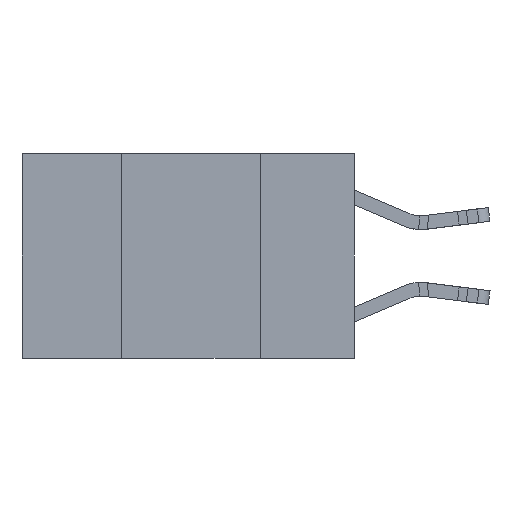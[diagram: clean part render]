
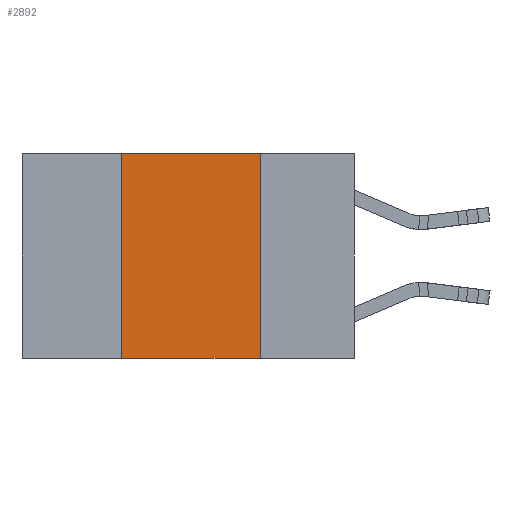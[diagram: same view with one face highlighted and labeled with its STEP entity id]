
A CAD part, left-side view. The second image highlights one B-rep face of the part: STEP entity #2892.
In plain terms, the highlighted planar face has unit normal (-1, 0, 0).
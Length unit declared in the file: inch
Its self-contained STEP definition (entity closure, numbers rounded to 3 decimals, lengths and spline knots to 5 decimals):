
#360 = LINE ( 'NONE', #27337, #17526 ) ;
#575 = LINE ( 'NONE', #24805, #24585 ) ;
#796 = CARTESIAN_POINT ( 'NONE',  ( 0., 0.17, -0.37 ) ) ;
#975 = VERTEX_POINT ( 'NONE', #23455 ) ;
#1849 = DIRECTION ( 'NONE',  ( 0., -1., 0. ) ) ;
#1882 = AXIS2_PLACEMENT_3D ( 'NONE', #5179, #29507, #25401 ) ;
#2091 = DIRECTION ( 'NONE',  ( 0., 0., 1. ) ) ;
#2797 = DIRECTION ( 'NONE',  ( 0., 0., -1. ) ) ;
#2892 = ADVANCED_FACE ( 'NONE', ( #9422 ), #16339, .F. ) ;
#4209 = VECTOR ( 'NONE', #2797, 39.37008 ) ;
#4938 = LINE ( 'NONE', #5196, #4209 ) ;
#5125 = CARTESIAN_POINT ( 'NONE',  ( 0., 0.17, 0. ) ) ;
#5179 = CARTESIAN_POINT ( 'NONE',  ( 0., 0.6, 0. ) ) ;
#5196 = CARTESIAN_POINT ( 'NONE',  ( 0., 0.17, 0. ) ) ;
#8936 = VERTEX_POINT ( 'NONE', #5125 ) ;
#9033 = VERTEX_POINT ( 'NONE', #796 ) ;
#9422 = FACE_OUTER_BOUND ( 'NONE', #16592, .T. ) ;
#9629 = EDGE_CURVE ( 'NONE', #8936, #9033, #4938, .T. ) ;
#10108 = ORIENTED_EDGE ( 'NONE', *, *, #12278, .F. ) ;
#12278 = EDGE_CURVE ( 'NONE', #975, #22771, #14289, .T. ) ;
#13565 = VECTOR ( 'NONE', #2091, 39.37008 ) ;
#13722 = ORIENTED_EDGE ( 'NONE', *, *, #23554, .F. ) ;
#13771 = CARTESIAN_POINT ( 'NONE',  ( 0., 0.42, 0. ) ) ;
#14289 = LINE ( 'NONE', #13771, #13565 ) ;
#16339 = PLANE ( 'NONE',  #1882 ) ;
#16592 = EDGE_LOOP ( 'NONE', ( #21715, #13722, #10108, #26394 ) ) ;
#17526 = VECTOR ( 'NONE', #1849, 39.37008 ) ;
#20168 = EDGE_CURVE ( 'NONE', #975, #9033, #575, .T. ) ;
#21715 = ORIENTED_EDGE ( 'NONE', *, *, #9629, .F. ) ;
#22771 = VERTEX_POINT ( 'NONE', #28849 ) ;
#23455 = CARTESIAN_POINT ( 'NONE',  ( 0., 0.42, -0.37 ) ) ;
#23554 = EDGE_CURVE ( 'NONE', #22771, #8936, #360, .T. ) ;
#24585 = VECTOR ( 'NONE', #27110, 39.37008 ) ;
#24805 = CARTESIAN_POINT ( 'NONE',  ( 0., 0.6, -0.37 ) ) ;
#25401 = DIRECTION ( 'NONE',  ( 0., 0., -1. ) ) ;
#26394 = ORIENTED_EDGE ( 'NONE', *, *, #20168, .T. ) ;
#27110 = DIRECTION ( 'NONE',  ( 0., -1., 0. ) ) ;
#27337 = CARTESIAN_POINT ( 'NONE',  ( 0., 0.6, 0. ) ) ;
#28849 = CARTESIAN_POINT ( 'NONE',  ( 0., 0.42, 0. ) ) ;
#29507 = DIRECTION ( 'NONE',  ( 1., 0., 0. ) ) ;
